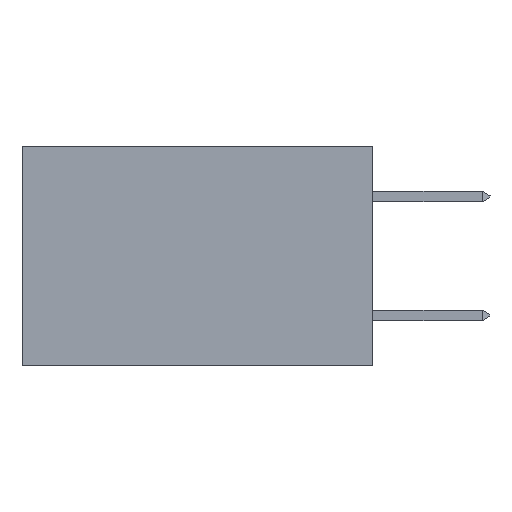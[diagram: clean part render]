
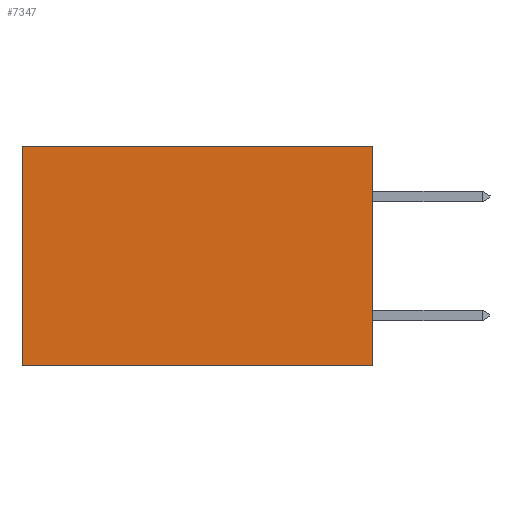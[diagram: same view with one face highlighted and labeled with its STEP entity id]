
A CAD part, left-side view. The second image highlights one B-rep face of the part: STEP entity #7347.
In plain terms, the highlighted planar face has unit normal (-1, 0, 0).
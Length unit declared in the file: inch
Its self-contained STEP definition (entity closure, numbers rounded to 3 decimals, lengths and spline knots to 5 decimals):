
#106 = DIRECTION ( 'NONE',  ( 0., 1., 0. ) ) ;
#519 = VERTEX_POINT ( 'NONE', #13831 ) ;
#969 = LINE ( 'NONE', #1259, #4925 ) ;
#1259 = CARTESIAN_POINT ( 'NONE',  ( 0.277, 0., -0.37 ) ) ;
#1776 = DIRECTION ( 'NONE',  ( 0., 1., 0. ) ) ;
#2937 = EDGE_CURVE ( 'NONE', #12653, #5176, #21111, .T. ) ;
#3117 = ORIENTED_EDGE ( 'NONE', *, *, #2937, .T. ) ;
#3332 = EDGE_CURVE ( 'NONE', #16627, #5176, #969, .T. ) ;
#3561 = VECTOR ( 'NONE', #106, 39.37008 ) ;
#4054 = EDGE_CURVE ( 'NONE', #519, #16627, #4627, .T. ) ;
#4627 = LINE ( 'NONE', #5057, #17480 ) ;
#4925 = VECTOR ( 'NONE', #1776, 39.37008 ) ;
#5057 = CARTESIAN_POINT ( 'NONE',  ( 0.277, 0., -0.37 ) ) ;
#5176 = VERTEX_POINT ( 'NONE', #7253 ) ;
#7253 = CARTESIAN_POINT ( 'NONE',  ( 0.277, 0.59, -0.37 ) ) ;
#7347 = ADVANCED_FACE ( 'NONE', ( #8086 ), #7587, .F. ) ;
#7581 = LINE ( 'NONE', #11990, #3561 ) ;
#7587 = PLANE ( 'NONE',  #16681 ) ;
#8086 = FACE_OUTER_BOUND ( 'NONE', #20913, .T. ) ;
#8559 = CARTESIAN_POINT ( 'NONE',  ( 0.277, 0.59, 0. ) ) ;
#10043 = DIRECTION ( 'NONE',  ( 0., 0., -1. ) ) ;
#10967 = DIRECTION ( 'NONE',  ( 0., 0., -1. ) ) ;
#11990 = CARTESIAN_POINT ( 'NONE',  ( 0.277, 0., 0. ) ) ;
#12653 = VERTEX_POINT ( 'NONE', #8559 ) ;
#13831 = CARTESIAN_POINT ( 'NONE',  ( 0.277, 0., 0. ) ) ;
#14319 = DIRECTION ( 'NONE',  ( 0., 0., -1. ) ) ;
#14456 = CARTESIAN_POINT ( 'NONE',  ( 0.277, 0.59, -0.37 ) ) ;
#16077 = ORIENTED_EDGE ( 'NONE', *, *, #17327, .T. ) ;
#16627 = VERTEX_POINT ( 'NONE', #17503 ) ;
#16681 = AXIS2_PLACEMENT_3D ( 'NONE', #19218, #20855, #10967 ) ;
#17327 = EDGE_CURVE ( 'NONE', #519, #12653, #7581, .T. ) ;
#17480 = VECTOR ( 'NONE', #10043, 39.37008 ) ;
#17503 = CARTESIAN_POINT ( 'NONE',  ( 0.277, 0., -0.37 ) ) ;
#18072 = ORIENTED_EDGE ( 'NONE', *, *, #3332, .F. ) ;
#19218 = CARTESIAN_POINT ( 'NONE',  ( 0.277, 0., -0.37 ) ) ;
#20855 = DIRECTION ( 'NONE',  ( 1., 0., 0. ) ) ;
#20873 = VECTOR ( 'NONE', #14319, 39.37008 ) ;
#20913 = EDGE_LOOP ( 'NONE', ( #3117, #18072, #21182, #16077 ) ) ;
#21111 = LINE ( 'NONE', #14456, #20873 ) ;
#21182 = ORIENTED_EDGE ( 'NONE', *, *, #4054, .F. ) ;
